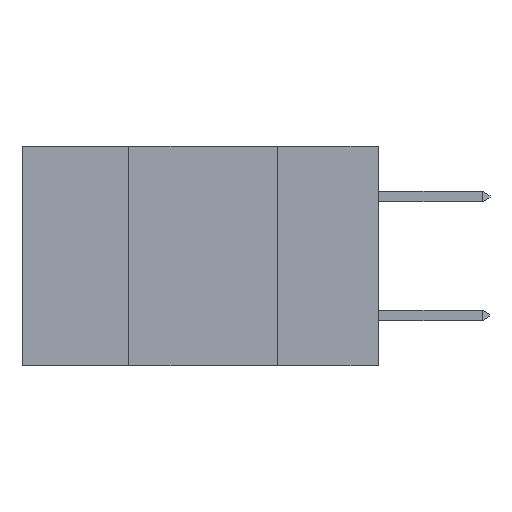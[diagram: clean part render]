
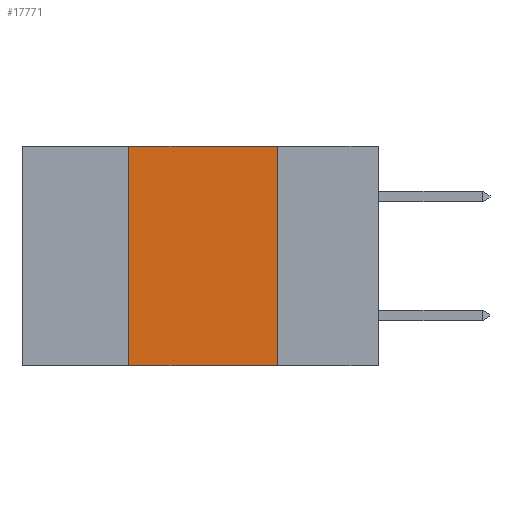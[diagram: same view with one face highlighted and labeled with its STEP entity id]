
A CAD part, left-side view. The second image highlights one B-rep face of the part: STEP entity #17771.
In plain terms, the highlighted planar face has unit normal (-1, 0, 0).
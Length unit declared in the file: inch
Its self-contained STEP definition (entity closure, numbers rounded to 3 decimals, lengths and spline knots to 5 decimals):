
#51 = DIRECTION ( 'NONE',  ( 0., -1., 0. ) ) ;
#1178 = CARTESIAN_POINT ( 'NONE',  ( 0., 0.6, 0. ) ) ;
#1427 = CARTESIAN_POINT ( 'NONE',  ( 0., 0.17, 0. ) ) ;
#1460 = EDGE_CURVE ( 'NONE', #10063, #14430, #13927, .T. ) ;
#1572 = ORIENTED_EDGE ( 'NONE', *, *, #1460, .T. ) ;
#1880 = EDGE_CURVE ( 'NONE', #14539, #2155, #15130, .T. ) ;
#2155 = VERTEX_POINT ( 'NONE', #1427 ) ;
#3805 = AXIS2_PLACEMENT_3D ( 'NONE', #14062, #15600, #6519 ) ;
#4180 = EDGE_LOOP ( 'NONE', ( #8884, #7219, #15129, #1572 ) ) ;
#4846 = CARTESIAN_POINT ( 'NONE',  ( 0., 0.17, -0.37 ) ) ;
#4984 = PLANE ( 'NONE',  #3805 ) ;
#5086 = CARTESIAN_POINT ( 'NONE',  ( 0., 0.17, 0. ) ) ;
#6519 = DIRECTION ( 'NONE',  ( 0., 0., -1. ) ) ;
#7073 = VECTOR ( 'NONE', #51, 39.37008 ) ;
#7219 = ORIENTED_EDGE ( 'NONE', *, *, #1880, .F. ) ;
#8439 = CARTESIAN_POINT ( 'NONE',  ( 0., 0.6, -0.37 ) ) ;
#8884 = ORIENTED_EDGE ( 'NONE', *, *, #16456, .F. ) ;
#9071 = DIRECTION ( 'NONE',  ( 0., -1., 0. ) ) ;
#9822 = VECTOR ( 'NONE', #9071, 39.37008 ) ;
#10063 = VERTEX_POINT ( 'NONE', #10728 ) ;
#10728 = CARTESIAN_POINT ( 'NONE',  ( 0., 0.42, -0.37 ) ) ;
#11040 = FACE_OUTER_BOUND ( 'NONE', #4180, .T. ) ;
#12615 = CARTESIAN_POINT ( 'NONE',  ( 0., 0.42, 0. ) ) ;
#13927 = LINE ( 'NONE', #8439, #9822 ) ;
#14062 = CARTESIAN_POINT ( 'NONE',  ( 0., 0.6, 0. ) ) ;
#14430 = VERTEX_POINT ( 'NONE', #4846 ) ;
#14539 = VERTEX_POINT ( 'NONE', #12615 ) ;
#14573 = LINE ( 'NONE', #17934, #18613 ) ;
#14864 = DIRECTION ( 'NONE',  ( 0., 0., 1. ) ) ;
#15129 = ORIENTED_EDGE ( 'NONE', *, *, #19909, .F. ) ;
#15130 = LINE ( 'NONE', #1178, #7073 ) ;
#15600 = DIRECTION ( 'NONE',  ( 1., 0., 0. ) ) ;
#15706 = DIRECTION ( 'NONE',  ( 0., 0., -1. ) ) ;
#16456 = EDGE_CURVE ( 'NONE', #2155, #14430, #18751, .T. ) ;
#17771 = ADVANCED_FACE ( 'NONE', ( #11040 ), #4984, .F. ) ;
#17934 = CARTESIAN_POINT ( 'NONE',  ( 0., 0.42, 0. ) ) ;
#18613 = VECTOR ( 'NONE', #14864, 39.37008 ) ;
#18751 = LINE ( 'NONE', #5086, #19198 ) ;
#19198 = VECTOR ( 'NONE', #15706, 39.37008 ) ;
#19909 = EDGE_CURVE ( 'NONE', #10063, #14539, #14573, .T. ) ;
